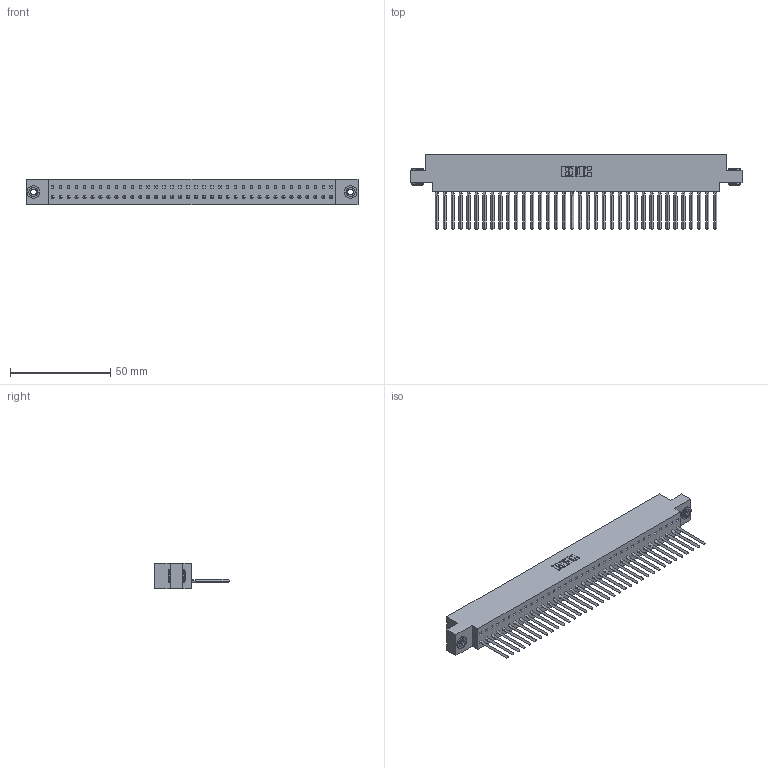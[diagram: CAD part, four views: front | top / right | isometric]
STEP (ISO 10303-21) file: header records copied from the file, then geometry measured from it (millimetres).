
FILE_DESCRIPTION (( 'STEP AP203' ), '1' );
FILE_NAME ('317-036-541-603.STEP', '2020-02-27T22:37:26', ( '' ), ( '' ), 'SwSTEP 2.0', 'SolidWorks 2016', '' );
FILE_SCHEMA (( 'CONFIG_CONTROL_DESIGN' ));
Length unit declared in the file: inch
Products named in the file (4): 317-290-002_541; 345-250-002_345-250-002-102; 317-036-541-603; 317 Part_.156 Dia - TH
Assembly tree (39 placements, depth 2):
  317-036-541-603
    317 Part_.156 Dia - TH
    317-290-002_541  x36
    345-250-002_345-250-002-102  x2
Bounding box: 165.35 x 37.34 x 12.7 mm (x, y, z)
Volume: 26649.8 mm3; surface area: 37672.6 mm2
Topology: 39 solids, 39 shells, 5612 faces, 15975 edges, 10382 vertices
Faces by surface type: plane 4532, cylinder 928, bspline 144, cone 8
Entity records: 53921 total; most frequent: CARTESIAN_POINT 10192, ORIENTED_EDGE 9474, DIRECTION 7819, EDGE_CURVE 4737, VECTOR 4349, LINE 4349, VERTEX_POINT 3148, AXIS2_PLACEMENT_3D 1735
